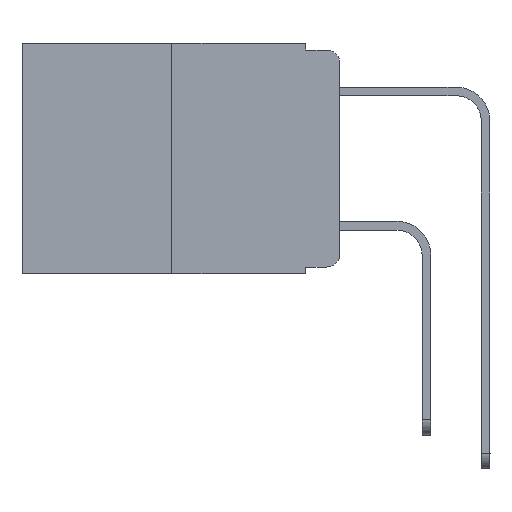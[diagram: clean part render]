
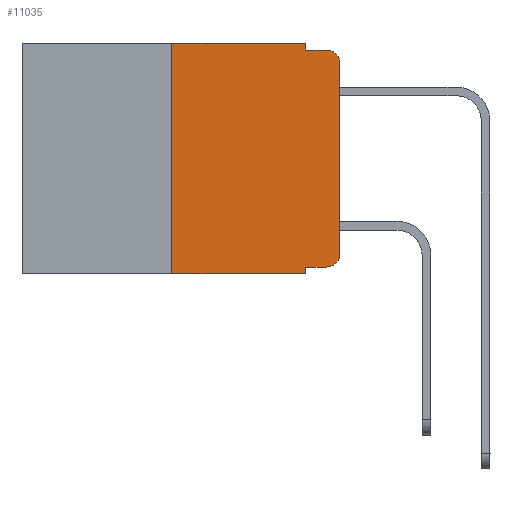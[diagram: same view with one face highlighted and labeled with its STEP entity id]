
A CAD part, left-side view. The second image highlights one B-rep face of the part: STEP entity #11035.
In plain terms, the highlighted planar face has unit normal (-1, 0, 0).
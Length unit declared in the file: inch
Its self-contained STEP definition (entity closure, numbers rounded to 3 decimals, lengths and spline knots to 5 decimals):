
#103 = DIRECTION ( 'NONE',  ( 0., -1., 0. ) ) ;
#322 = CARTESIAN_POINT ( 'NONE',  ( 0., 0.051, -0.343 ) ) ;
#863 = LINE ( 'NONE', #6469, #15782 ) ;
#1046 = CARTESIAN_POINT ( 'NONE',  ( 0., 0.25, 0. ) ) ;
#1170 = CARTESIAN_POINT ( 'NONE',  ( 0., 0.051, -0.01 ) ) ;
#1215 = ORIENTED_EDGE ( 'NONE', *, *, #13396, .T. ) ;
#1251 = EDGE_CURVE ( 'NONE', #6510, #7393, #5377, .T. ) ;
#1309 = DIRECTION ( 'NONE',  ( 0., 0., -1. ) ) ;
#1312 = CARTESIAN_POINT ( 'NONE',  ( 0., 0.02, -0.03 ) ) ;
#1445 = CIRCLE ( 'NONE', #3659, 0.02 ) ;
#2437 = CARTESIAN_POINT ( 'NONE',  ( 0., 0.051, 0. ) ) ;
#2695 = CARTESIAN_POINT ( 'NONE',  ( 0., 0.02, -0.313 ) ) ;
#2802 = VECTOR ( 'NONE', #12866, 39.37008 ) ;
#3136 = VERTEX_POINT ( 'NONE', #6053 ) ;
#3330 = VERTEX_POINT ( 'NONE', #14313 ) ;
#3398 = DIRECTION ( 'NONE',  ( 0., 0., -1. ) ) ;
#3480 = DIRECTION ( 'NONE',  ( 1., 0., 0. ) ) ;
#3659 = AXIS2_PLACEMENT_3D ( 'NONE', #1312, #5369, #6341 ) ;
#3698 = VERTEX_POINT ( 'NONE', #15761 ) ;
#4325 = CARTESIAN_POINT ( 'NONE',  ( 0., 0., -0.03 ) ) ;
#4546 = EDGE_CURVE ( 'NONE', #6510, #15818, #9083, .T. ) ;
#5027 = CARTESIAN_POINT ( 'NONE',  ( 0., 0.051, 0. ) ) ;
#5187 = DIRECTION ( 'NONE',  ( -1., 0., 0. ) ) ;
#5201 = LINE ( 'NONE', #14256, #15091 ) ;
#5216 = VERTEX_POINT ( 'NONE', #13433 ) ;
#5218 = ORIENTED_EDGE ( 'NONE', *, *, #10045, .F. ) ;
#5349 = CARTESIAN_POINT ( 'NONE',  ( 0., 0.051, -0.333 ) ) ;
#5369 = DIRECTION ( 'NONE',  ( -1., 0., 0. ) ) ;
#5377 = LINE ( 'NONE', #10314, #9021 ) ;
#5471 = VERTEX_POINT ( 'NONE', #13337 ) ;
#5542 = DIRECTION ( 'NONE',  ( 0., 0., -1. ) ) ;
#5845 = EDGE_CURVE ( 'NONE', #8324, #5216, #1445, .T. ) ;
#6053 = CARTESIAN_POINT ( 'NONE',  ( 0., 0.051, 0. ) ) ;
#6247 = EDGE_LOOP ( 'NONE', ( #11908, #14727, #12162, #7263, #5218, #13631, #12427, #9948, #9307, #1215 ) ) ;
#6341 = DIRECTION ( 'NONE',  ( 0., 0., -1. ) ) ;
#6469 = CARTESIAN_POINT ( 'NONE',  ( 0., 0.473, -0.343 ) ) ;
#6510 = VERTEX_POINT ( 'NONE', #5349 ) ;
#6584 = VECTOR ( 'NONE', #13141, 39.37008 ) ;
#7099 = FACE_OUTER_BOUND ( 'NONE', #6247, .T. ) ;
#7137 = VECTOR ( 'NONE', #16841, 39.37008 ) ;
#7263 = ORIENTED_EDGE ( 'NONE', *, *, #11275, .F. ) ;
#7393 = VERTEX_POINT ( 'NONE', #13397 ) ;
#8256 = EDGE_CURVE ( 'NONE', #9058, #5216, #5201, .T. ) ;
#8324 = VERTEX_POINT ( 'NONE', #4325 ) ;
#9021 = VECTOR ( 'NONE', #14438, 39.37008 ) ;
#9058 = VERTEX_POINT ( 'NONE', #1170 ) ;
#9071 = LINE ( 'NONE', #5027, #6584 ) ;
#9083 = LINE ( 'NONE', #2437, #9347 ) ;
#9307 = ORIENTED_EDGE ( 'NONE', *, *, #1251, .T. ) ;
#9347 = VECTOR ( 'NONE', #1309, 39.37008 ) ;
#9948 = ORIENTED_EDGE ( 'NONE', *, *, #4546, .F. ) ;
#10045 = EDGE_CURVE ( 'NONE', #5471, #3136, #11917, .T. ) ;
#10314 = CARTESIAN_POINT ( 'NONE',  ( 0., 0.051, -0.333 ) ) ;
#10356 = LINE ( 'NONE', #15446, #2802 ) ;
#10700 = AXIS2_PLACEMENT_3D ( 'NONE', #15673, #3480, #3398 ) ;
#11035 = ADVANCED_FACE ( 'NONE', ( #7099 ), #12374, .F. ) ;
#11275 = EDGE_CURVE ( 'NONE', #3136, #9058, #9071, .T. ) ;
#11908 = ORIENTED_EDGE ( 'NONE', *, *, #15064, .T. ) ;
#11917 = LINE ( 'NONE', #14497, #16733 ) ;
#12162 = ORIENTED_EDGE ( 'NONE', *, *, #8256, .F. ) ;
#12374 = PLANE ( 'NONE',  #10700 ) ;
#12395 = CIRCLE ( 'NONE', #12681, 0.02 ) ;
#12427 = ORIENTED_EDGE ( 'NONE', *, *, #16950, .T. ) ;
#12681 = AXIS2_PLACEMENT_3D ( 'NONE', #2695, #5187, #5542 ) ;
#12781 = DIRECTION ( 'NONE',  ( 0., -1., 0. ) ) ;
#12866 = DIRECTION ( 'NONE',  ( 0., 0., 1. ) ) ;
#12979 = LINE ( 'NONE', #1046, #7137 ) ;
#13141 = DIRECTION ( 'NONE',  ( 0., 0., -1. ) ) ;
#13236 = EDGE_CURVE ( 'NONE', #3330, #5471, #12979, .T. ) ;
#13337 = CARTESIAN_POINT ( 'NONE',  ( 0., 0.25, 0. ) ) ;
#13396 = EDGE_CURVE ( 'NONE', #7393, #3698, #12395, .T. ) ;
#13397 = CARTESIAN_POINT ( 'NONE',  ( 0., 0.02, -0.333 ) ) ;
#13433 = CARTESIAN_POINT ( 'NONE',  ( 0., 0.02, -0.01 ) ) ;
#13631 = ORIENTED_EDGE ( 'NONE', *, *, #13236, .F. ) ;
#14256 = CARTESIAN_POINT ( 'NONE',  ( 0., 0.051, -0.01 ) ) ;
#14313 = CARTESIAN_POINT ( 'NONE',  ( 0., 0.25, -0.343 ) ) ;
#14438 = DIRECTION ( 'NONE',  ( 0., -1., 0. ) ) ;
#14497 = CARTESIAN_POINT ( 'NONE',  ( 0., 0.473, 0. ) ) ;
#14727 = ORIENTED_EDGE ( 'NONE', *, *, #5845, .T. ) ;
#15064 = EDGE_CURVE ( 'NONE', #3698, #8324, #10356, .T. ) ;
#15091 = VECTOR ( 'NONE', #15730, 39.37008 ) ;
#15446 = CARTESIAN_POINT ( 'NONE',  ( 0., 0., 0. ) ) ;
#15673 = CARTESIAN_POINT ( 'NONE',  ( 0., 0.473, 0. ) ) ;
#15730 = DIRECTION ( 'NONE',  ( 0., -1., 0. ) ) ;
#15761 = CARTESIAN_POINT ( 'NONE',  ( 0., 0., -0.313 ) ) ;
#15782 = VECTOR ( 'NONE', #12781, 39.37008 ) ;
#15818 = VERTEX_POINT ( 'NONE', #322 ) ;
#16733 = VECTOR ( 'NONE', #103, 39.37008 ) ;
#16841 = DIRECTION ( 'NONE',  ( 0., 0., 1. ) ) ;
#16950 = EDGE_CURVE ( 'NONE', #3330, #15818, #863, .T. ) ;
